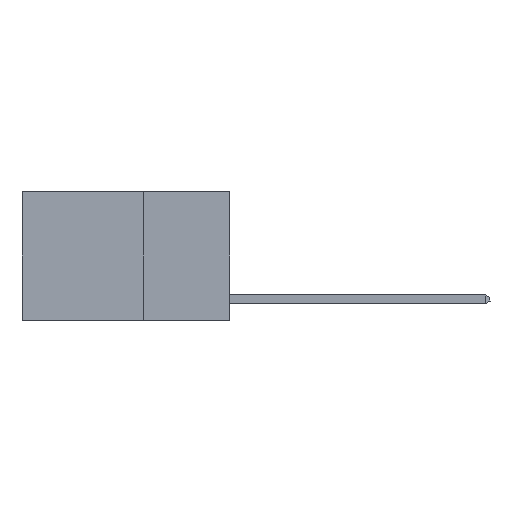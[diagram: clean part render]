
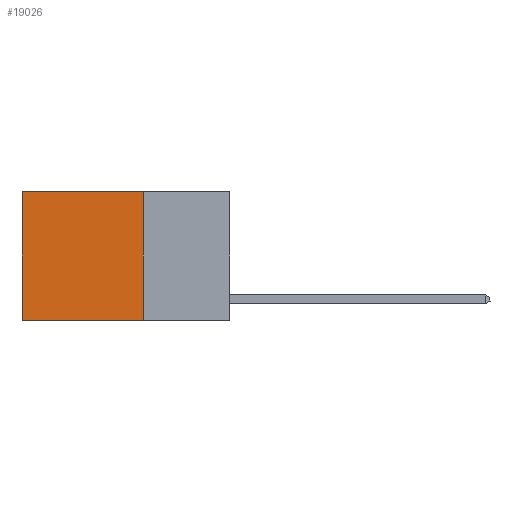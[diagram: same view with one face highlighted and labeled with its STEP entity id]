
A CAD part, left-side view. The second image highlights one B-rep face of the part: STEP entity #19026.
In plain terms, the highlighted planar face has unit normal (-1, 0, 0).
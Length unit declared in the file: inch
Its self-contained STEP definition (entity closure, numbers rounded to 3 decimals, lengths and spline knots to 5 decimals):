
#590 = CARTESIAN_POINT ( 'NONE',  ( 0.2625, 0.25, -0.37 ) ) ;
#787 = VERTEX_POINT ( 'NONE', #15537 ) ;
#1280 = ORIENTED_EDGE ( 'NONE', *, *, #10831, .T. ) ;
#1548 = LINE ( 'NONE', #21363, #20433 ) ;
#2256 = FACE_OUTER_BOUND ( 'NONE', #9305, .T. ) ;
#3859 = PLANE ( 'NONE',  #6843 ) ;
#5868 = VECTOR ( 'NONE', #15229, 39.37008 ) ;
#6538 = VERTEX_POINT ( 'NONE', #590 ) ;
#6843 = AXIS2_PLACEMENT_3D ( 'NONE', #9378, #7612, #20302 ) ;
#7612 = DIRECTION ( 'NONE',  ( 1., 0., 0. ) ) ;
#8645 = LINE ( 'NONE', #18655, #17760 ) ;
#8962 = LINE ( 'NONE', #17329, #22214 ) ;
#9305 = EDGE_LOOP ( 'NONE', ( #12120, #17090, #9516, #1280 ) ) ;
#9378 = CARTESIAN_POINT ( 'NONE',  ( 0.2625, 0.25, 0. ) ) ;
#9516 = ORIENTED_EDGE ( 'NONE', *, *, #19082, .F. ) ;
#10151 = CARTESIAN_POINT ( 'NONE',  ( 0.2625, 0.6, 0. ) ) ;
#10831 = EDGE_CURVE ( 'NONE', #787, #17975, #8962, .T. ) ;
#12120 = ORIENTED_EDGE ( 'NONE', *, *, #21962, .T. ) ;
#13420 = CARTESIAN_POINT ( 'NONE',  ( 0.2625, 0.6, 0. ) ) ;
#14227 = DIRECTION ( 'NONE',  ( 0., 1., 0. ) ) ;
#14276 = CARTESIAN_POINT ( 'NONE',  ( 0.2625, 0.6, -0.37 ) ) ;
#14536 = EDGE_CURVE ( 'NONE', #6538, #20111, #1548, .T. ) ;
#15229 = DIRECTION ( 'NONE',  ( 0., 0., -1. ) ) ;
#15537 = CARTESIAN_POINT ( 'NONE',  ( 0.2625, 0.25, 0. ) ) ;
#15584 = DIRECTION ( 'NONE',  ( 0., 1., 0. ) ) ;
#15620 = LINE ( 'NONE', #13420, #5868 ) ;
#17090 = ORIENTED_EDGE ( 'NONE', *, *, #14536, .F. ) ;
#17329 = CARTESIAN_POINT ( 'NONE',  ( 0.2625, 0.25, 0. ) ) ;
#17760 = VECTOR ( 'NONE', #20455, 39.37008 ) ;
#17975 = VERTEX_POINT ( 'NONE', #10151 ) ;
#18655 = CARTESIAN_POINT ( 'NONE',  ( 0.2625, 0.25, 0. ) ) ;
#19026 = ADVANCED_FACE ( 'NONE', ( #2256 ), #3859, .F. ) ;
#19082 = EDGE_CURVE ( 'NONE', #787, #6538, #8645, .T. ) ;
#20111 = VERTEX_POINT ( 'NONE', #14276 ) ;
#20302 = DIRECTION ( 'NONE',  ( 0., 0., -1. ) ) ;
#20433 = VECTOR ( 'NONE', #14227, 39.37008 ) ;
#20455 = DIRECTION ( 'NONE',  ( 0., 0., -1. ) ) ;
#21363 = CARTESIAN_POINT ( 'NONE',  ( 0.2625, 0.25, -0.37 ) ) ;
#21962 = EDGE_CURVE ( 'NONE', #17975, #20111, #15620, .T. ) ;
#22214 = VECTOR ( 'NONE', #15584, 39.37008 ) ;
